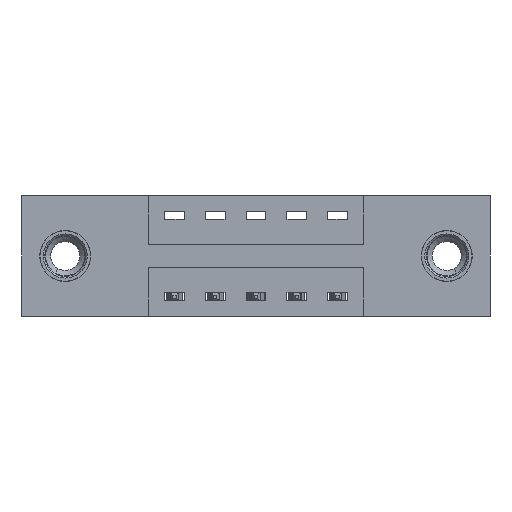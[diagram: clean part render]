
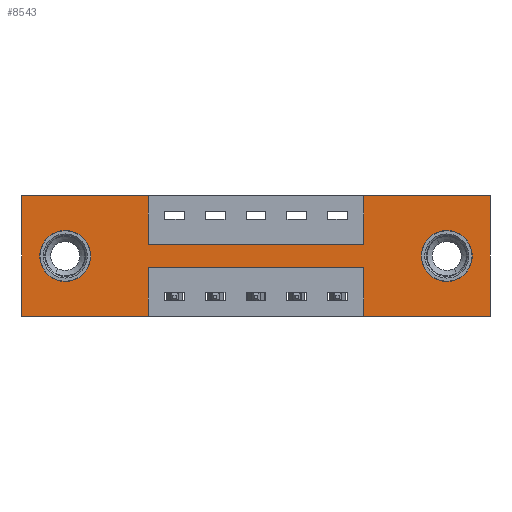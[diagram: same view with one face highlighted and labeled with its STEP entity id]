
A CAD part, front view. The second image highlights one B-rep face of the part: STEP entity #8543.
In plain terms, the highlighted planar face has unit normal (0, -1, 0).
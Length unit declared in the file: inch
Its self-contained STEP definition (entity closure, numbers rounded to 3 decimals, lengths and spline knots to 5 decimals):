
#22 = VECTOR ( 'NONE', #8490, 39.37008 ) ;
#75 = VERTEX_POINT ( 'NONE', #1835 ) ;
#184 = ORIENTED_EDGE ( 'NONE', *, *, #836, .F. ) ;
#211 = ORIENTED_EDGE ( 'NONE', *, *, #6784, .F. ) ;
#266 = VERTEX_POINT ( 'NONE', #9153 ) ;
#317 = EDGE_CURVE ( 'NONE', #266, #2327, #2541, .T. ) ;
#367 = ORIENTED_EDGE ( 'NONE', *, *, #10353, .F. ) ;
#428 = EDGE_CURVE ( 'NONE', #75, #11007, #4970, .T. ) ;
#526 = CARTESIAN_POINT ( 'NONE',  ( 0., 0., 0. ) ) ;
#573 = ORIENTED_EDGE ( 'NONE', *, *, #4342, .F. ) ;
#660 = LINE ( 'NONE', #12296, #22 ) ;
#707 = AXIS2_PLACEMENT_3D ( 'NONE', #7121, #3162, #4424 ) ;
#780 = VERTEX_POINT ( 'NONE', #3650 ) ;
#809 = DIRECTION ( 'NONE',  ( 0., 0., 1. ) ) ;
#836 = EDGE_CURVE ( 'NONE', #11123, #12617, #5422, .T. ) ;
#872 = CARTESIAN_POINT ( 'NONE',  ( 1.0475, 0., -0.37 ) ) ;
#898 = FACE_OUTER_BOUND ( 'NONE', #12749, .T. ) ;
#903 = ORIENTED_EDGE ( 'NONE', *, *, #4126, .F. ) ;
#985 = CARTESIAN_POINT ( 'NONE',  ( 0.3875, 0., 0. ) ) ;
#1027 = DIRECTION ( 'NONE',  ( 0., 0., -1. ) ) ;
#1268 = CARTESIAN_POINT ( 'NONE',  ( 1.3025, 0., -0.107 ) ) ;
#1344 = VECTOR ( 'NONE', #5970, 39.37008 ) ;
#1497 = ORIENTED_EDGE ( 'NONE', *, *, #428, .F. ) ;
#1562 = LINE ( 'NONE', #2138, #7962 ) ;
#1754 = LINE ( 'NONE', #526, #5614 ) ;
#1806 = ORIENTED_EDGE ( 'NONE', *, *, #317, .T. ) ;
#1835 = CARTESIAN_POINT ( 'NONE',  ( 0., 0., 0. ) ) ;
#1895 = VECTOR ( 'NONE', #11342, 39.37008 ) ;
#1933 = DIRECTION ( 'NONE',  ( 0., 0., 1. ) ) ;
#2132 = EDGE_CURVE ( 'NONE', #12617, #12692, #1754, .T. ) ;
#2138 = CARTESIAN_POINT ( 'NONE',  ( 0., 0., -0.37 ) ) ;
#2327 = VERTEX_POINT ( 'NONE', #1268 ) ;
#2353 = CARTESIAN_POINT ( 'NONE',  ( 0.3875, 0., -0.37 ) ) ;
#2398 = CARTESIAN_POINT ( 'NONE',  ( 1.3025, 0., -0.185 ) ) ;
#2541 = CIRCLE ( 'NONE', #12313, 0.078 ) ;
#2700 = DIRECTION ( 'NONE',  ( 0., 0., 1. ) ) ;
#2710 = DIRECTION ( 'NONE',  ( 0., 0., -1. ) ) ;
#2862 = CARTESIAN_POINT ( 'NONE',  ( 1.0475, 0., 0. ) ) ;
#2961 = VERTEX_POINT ( 'NONE', #12538 ) ;
#3001 = ORIENTED_EDGE ( 'NONE', *, *, #3483, .T. ) ;
#3076 = ORIENTED_EDGE ( 'NONE', *, *, #7315, .F. ) ;
#3162 = DIRECTION ( 'NONE',  ( 0., -1., 0. ) ) ;
#3384 = ORIENTED_EDGE ( 'NONE', *, *, #2132, .F. ) ;
#3483 = EDGE_CURVE ( 'NONE', #780, #7827, #10088, .T. ) ;
#3493 = VECTOR ( 'NONE', #7335, 39.37008 ) ;
#3505 = ORIENTED_EDGE ( 'NONE', *, *, #4901, .F. ) ;
#3650 = CARTESIAN_POINT ( 'NONE',  ( 0.1325, 0., -0.263 ) ) ;
#3716 = CIRCLE ( 'NONE', #10472, 0.078 ) ;
#4020 = CARTESIAN_POINT ( 'NONE',  ( 1.435, 0., 0. ) ) ;
#4087 = VECTOR ( 'NONE', #8999, 39.37008 ) ;
#4126 = EDGE_CURVE ( 'NONE', #12692, #7276, #8475, .T. ) ;
#4161 = AXIS2_PLACEMENT_3D ( 'NONE', #9097, #10112, #2710 ) ;
#4172 = VECTOR ( 'NONE', #8825, 39.37008 ) ;
#4228 = AXIS2_PLACEMENT_3D ( 'NONE', #7765, #8635, #2700 ) ;
#4342 = EDGE_CURVE ( 'NONE', #2961, #75, #5951, .T. ) ;
#4385 = CIRCLE ( 'NONE', #4161, 0.078 ) ;
#4424 = DIRECTION ( 'NONE',  ( 0., 0., -1. ) ) ;
#4551 = VERTEX_POINT ( 'NONE', #9969 ) ;
#4766 = CARTESIAN_POINT ( 'NONE',  ( 1.0475, 0., 0. ) ) ;
#4856 = CARTESIAN_POINT ( 'NONE',  ( 0.3875, 0., -0.15 ) ) ;
#4901 = EDGE_CURVE ( 'NONE', #12873, #2961, #1562, .T. ) ;
#4970 = LINE ( 'NONE', #9383, #1895 ) ;
#5356 = DIRECTION ( 'NONE',  ( -1., 0., 0. ) ) ;
#5422 = LINE ( 'NONE', #2862, #8558 ) ;
#5595 = VERTEX_POINT ( 'NONE', #5839 ) ;
#5614 = VECTOR ( 'NONE', #12351, 39.37008 ) ;
#5628 = LINE ( 'NONE', #12269, #12037 ) ;
#5632 = CARTESIAN_POINT ( 'NONE',  ( 1.435, 0., 0. ) ) ;
#5839 = CARTESIAN_POINT ( 'NONE',  ( 0.3875, 0., -0.15 ) ) ;
#5951 = LINE ( 'NONE', #7847, #10341 ) ;
#5954 = DIRECTION ( 'NONE',  ( -1., 0., 0. ) ) ;
#5970 = DIRECTION ( 'NONE',  ( 1., 0., 0. ) ) ;
#6010 = CARTESIAN_POINT ( 'NONE',  ( 1.0475, 0., -0.37 ) ) ;
#6095 = LINE ( 'NONE', #8957, #4087 ) ;
#6268 = EDGE_CURVE ( 'NONE', #7306, #12873, #6095, .T. ) ;
#6309 = CARTESIAN_POINT ( 'NONE',  ( 0.3875, 0., -0.22 ) ) ;
#6327 = VERTEX_POINT ( 'NONE', #6010 ) ;
#6460 = EDGE_CURVE ( 'NONE', #11007, #5595, #8921, .T. ) ;
#6508 = EDGE_CURVE ( 'NONE', #2327, #266, #4385, .T. ) ;
#6784 = EDGE_CURVE ( 'NONE', #4551, #7306, #5628, .T. ) ;
#6969 = ORIENTED_EDGE ( 'NONE', *, *, #11722, .T. ) ;
#6987 = ORIENTED_EDGE ( 'NONE', *, *, #11778, .F. ) ;
#7121 = CARTESIAN_POINT ( 'NONE',  ( 0., 0., -0.37 ) ) ;
#7212 = VECTOR ( 'NONE', #1027, 39.37008 ) ;
#7276 = VERTEX_POINT ( 'NONE', #8358 ) ;
#7306 = VERTEX_POINT ( 'NONE', #6309 ) ;
#7314 = DIRECTION ( 'NONE',  ( 0., 1., 0. ) ) ;
#7315 = EDGE_CURVE ( 'NONE', #7276, #6327, #660, .T. ) ;
#7335 = DIRECTION ( 'NONE',  ( 0., 0., -1. ) ) ;
#7403 = PLANE ( 'NONE',  #707 ) ;
#7738 = EDGE_LOOP ( 'NONE', ( #10260, #1806 ) ) ;
#7752 = EDGE_LOOP ( 'NONE', ( #6969, #3001 ) ) ;
#7765 = CARTESIAN_POINT ( 'NONE',  ( 0.1325, 0., -0.185 ) ) ;
#7827 = VERTEX_POINT ( 'NONE', #10391 ) ;
#7847 = CARTESIAN_POINT ( 'NONE',  ( 0., 0., 0. ) ) ;
#7962 = VECTOR ( 'NONE', #5954, 39.37008 ) ;
#8358 = CARTESIAN_POINT ( 'NONE',  ( 1.435, 0., -0.37 ) ) ;
#8475 = LINE ( 'NONE', #4020, #3493 ) ;
#8490 = DIRECTION ( 'NONE',  ( -1., 0., 0. ) ) ;
#8493 = ORIENTED_EDGE ( 'NONE', *, *, #6460, .F. ) ;
#8512 = FACE_BOUND ( 'NONE', #7738, .T. ) ;
#8543 = ADVANCED_FACE ( 'NONE', ( #8512, #8830, #898 ), #7403, .T. ) ;
#8558 = VECTOR ( 'NONE', #809, 39.37008 ) ;
#8635 = DIRECTION ( 'NONE',  ( 0., 1., 0. ) ) ;
#8825 = DIRECTION ( 'NONE',  ( 0., 0., 1. ) ) ;
#8830 = FACE_BOUND ( 'NONE', #7752, .T. ) ;
#8921 = LINE ( 'NONE', #985, #7212 ) ;
#8957 = CARTESIAN_POINT ( 'NONE',  ( 0.3875, 0., -0.37 ) ) ;
#8999 = DIRECTION ( 'NONE',  ( 0., 0., -1. ) ) ;
#9097 = CARTESIAN_POINT ( 'NONE',  ( 1.3025, 0., -0.185 ) ) ;
#9153 = CARTESIAN_POINT ( 'NONE',  ( 1.3025, 0., -0.263 ) ) ;
#9383 = CARTESIAN_POINT ( 'NONE',  ( 0., 0., 0. ) ) ;
#9457 = LINE ( 'NONE', #872, #4172 ) ;
#9732 = DIRECTION ( 'NONE',  ( 0., 0., 1. ) ) ;
#9836 = CARTESIAN_POINT ( 'NONE',  ( 0.1325, 0., -0.185 ) ) ;
#9969 = CARTESIAN_POINT ( 'NONE',  ( 1.0475, 0., -0.22 ) ) ;
#10088 = CIRCLE ( 'NONE', #4228, 0.078 ) ;
#10112 = DIRECTION ( 'NONE',  ( 0., 1., 0. ) ) ;
#10260 = ORIENTED_EDGE ( 'NONE', *, *, #6508, .T. ) ;
#10341 = VECTOR ( 'NONE', #9732, 39.37008 ) ;
#10353 = EDGE_CURVE ( 'NONE', #6327, #4551, #9457, .T. ) ;
#10391 = CARTESIAN_POINT ( 'NONE',  ( 0.1325, 0., -0.107 ) ) ;
#10472 = AXIS2_PLACEMENT_3D ( 'NONE', #9836, #10989, #1933 ) ;
#10989 = DIRECTION ( 'NONE',  ( 0., 1., 0. ) ) ;
#11007 = VERTEX_POINT ( 'NONE', #12547 ) ;
#11123 = VERTEX_POINT ( 'NONE', #11539 ) ;
#11300 = ORIENTED_EDGE ( 'NONE', *, *, #6268, .F. ) ;
#11342 = DIRECTION ( 'NONE',  ( 1., 0., 0. ) ) ;
#11539 = CARTESIAN_POINT ( 'NONE',  ( 1.0475, 0., -0.15 ) ) ;
#11722 = EDGE_CURVE ( 'NONE', #7827, #780, #3716, .T. ) ;
#11778 = EDGE_CURVE ( 'NONE', #5595, #11123, #12709, .T. ) ;
#12037 = VECTOR ( 'NONE', #5356, 39.37008 ) ;
#12269 = CARTESIAN_POINT ( 'NONE',  ( 0.3875, 0., -0.22 ) ) ;
#12296 = CARTESIAN_POINT ( 'NONE',  ( 0., 0., -0.37 ) ) ;
#12313 = AXIS2_PLACEMENT_3D ( 'NONE', #2398, #7314, #12336 ) ;
#12336 = DIRECTION ( 'NONE',  ( 0., 0., -1. ) ) ;
#12351 = DIRECTION ( 'NONE',  ( 1., 0., 0. ) ) ;
#12538 = CARTESIAN_POINT ( 'NONE',  ( 0., 0., -0.37 ) ) ;
#12547 = CARTESIAN_POINT ( 'NONE',  ( 0.3875, 0., 0. ) ) ;
#12617 = VERTEX_POINT ( 'NONE', #4766 ) ;
#12692 = VERTEX_POINT ( 'NONE', #5632 ) ;
#12709 = LINE ( 'NONE', #4856, #1344 ) ;
#12749 = EDGE_LOOP ( 'NONE', ( #11300, #211, #367, #3076, #903, #3384, #184, #6987, #8493, #1497, #573, #3505 ) ) ;
#12873 = VERTEX_POINT ( 'NONE', #2353 ) ;
